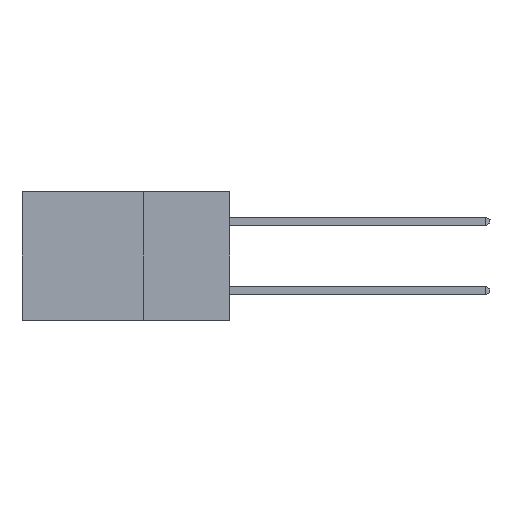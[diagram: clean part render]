
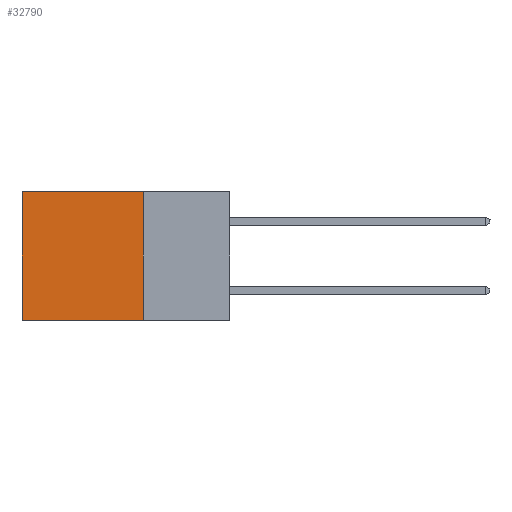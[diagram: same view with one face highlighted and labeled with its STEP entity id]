
A CAD part, left-side view. The second image highlights one B-rep face of the part: STEP entity #32790.
In plain terms, the highlighted planar face has unit normal (-1, 0, 0).
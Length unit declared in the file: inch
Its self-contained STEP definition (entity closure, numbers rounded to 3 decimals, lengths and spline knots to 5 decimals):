
#18 = LINE ( 'NONE', #20033, #19831 ) ;
#1696 = DIRECTION ( 'NONE',  ( 0., 1., 0. ) ) ;
#2334 = CARTESIAN_POINT ( 'NONE',  ( 0.298, 0.6, 0. ) ) ;
#2536 = ORIENTED_EDGE ( 'NONE', *, *, #11191, .F. ) ;
#3602 = EDGE_CURVE ( 'NONE', #13240, #24579, #29773, .T. ) ;
#4309 = CARTESIAN_POINT ( 'NONE',  ( 0.298, 0.25, 0. ) ) ;
#4934 = DIRECTION ( 'NONE',  ( 0., 0., -1. ) ) ;
#5109 = DIRECTION ( 'NONE',  ( 1., 0., 0. ) ) ;
#9449 = VECTOR ( 'NONE', #28956, 39.37008 ) ;
#9495 = FACE_OUTER_BOUND ( 'NONE', #25662, .T. ) ;
#9682 = CARTESIAN_POINT ( 'NONE',  ( 0.298, 0.6, -0.37 ) ) ;
#11017 = VECTOR ( 'NONE', #4934, 39.37008 ) ;
#11191 = EDGE_CURVE ( 'NONE', #32322, #13240, #18, .T. ) ;
#12655 = EDGE_CURVE ( 'NONE', #20870, #24579, #31292, .T. ) ;
#13240 = VERTEX_POINT ( 'NONE', #23851 ) ;
#14247 = VECTOR ( 'NONE', #1696, 39.37008 ) ;
#18662 = CARTESIAN_POINT ( 'NONE',  ( 0.298, 0.25, 0. ) ) ;
#18916 = AXIS2_PLACEMENT_3D ( 'NONE', #25521, #5109, #23117 ) ;
#19831 = VECTOR ( 'NONE', #32595, 39.37008 ) ;
#20033 = CARTESIAN_POINT ( 'NONE',  ( 0.298, 0.25, 0. ) ) ;
#20559 = PLANE ( 'NONE',  #18916 ) ;
#20689 = ORIENTED_EDGE ( 'NONE', *, *, #12655, .T. ) ;
#20870 = VERTEX_POINT ( 'NONE', #28830 ) ;
#21356 = CARTESIAN_POINT ( 'NONE',  ( 0.298, 0.25, -0.37 ) ) ;
#22315 = ORIENTED_EDGE ( 'NONE', *, *, #28421, .T. ) ;
#23117 = DIRECTION ( 'NONE',  ( 0., 0., -1. ) ) ;
#23851 = CARTESIAN_POINT ( 'NONE',  ( 0.298, 0.25, -0.37 ) ) ;
#24579 = VERTEX_POINT ( 'NONE', #9682 ) ;
#25223 = ORIENTED_EDGE ( 'NONE', *, *, #3602, .F. ) ;
#25521 = CARTESIAN_POINT ( 'NONE',  ( 0.298, 0.25, 0. ) ) ;
#25662 = EDGE_LOOP ( 'NONE', ( #20689, #25223, #2536, #22315 ) ) ;
#27710 = LINE ( 'NONE', #4309, #14247 ) ;
#28421 = EDGE_CURVE ( 'NONE', #32322, #20870, #27710, .T. ) ;
#28830 = CARTESIAN_POINT ( 'NONE',  ( 0.298, 0.6, 0. ) ) ;
#28956 = DIRECTION ( 'NONE',  ( 0., 1., 0. ) ) ;
#29773 = LINE ( 'NONE', #21356, #9449 ) ;
#31292 = LINE ( 'NONE', #2334, #11017 ) ;
#32322 = VERTEX_POINT ( 'NONE', #18662 ) ;
#32595 = DIRECTION ( 'NONE',  ( 0., 0., -1. ) ) ;
#32790 = ADVANCED_FACE ( 'NONE', ( #9495 ), #20559, .F. ) ;
